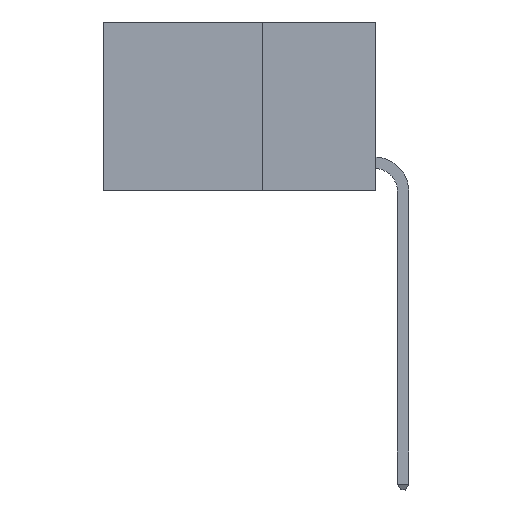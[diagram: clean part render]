
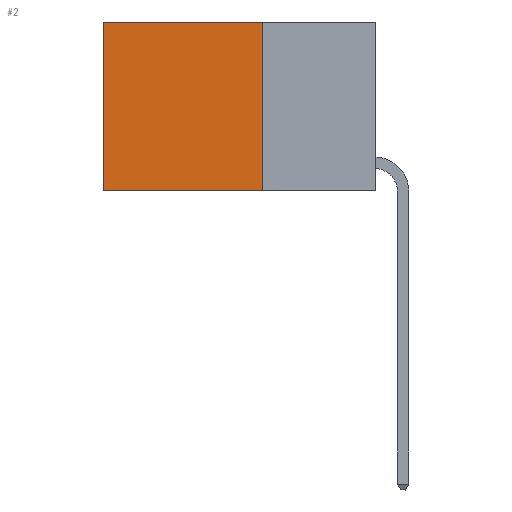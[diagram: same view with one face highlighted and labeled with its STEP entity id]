
A CAD part, left-side view. The second image highlights one B-rep face of the part: STEP entity #2.
In plain terms, the highlighted planar face has unit normal (-1, 0, 0).
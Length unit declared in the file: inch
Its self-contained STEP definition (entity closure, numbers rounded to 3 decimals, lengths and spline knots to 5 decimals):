
#2 = ADVANCED_FACE ( 'NONE', ( #24135 ), #3271, .F. ) ;
#2977 = EDGE_CURVE ( 'NONE', #5041, #15713, #22071, .T. ) ;
#3009 = EDGE_CURVE ( 'NONE', #5041, #8634, #20751, .T. ) ;
#3122 = CARTESIAN_POINT ( 'NONE',  ( 0.2625, 0.6, 0. ) ) ;
#3271 = PLANE ( 'NONE',  #3930 ) ;
#3333 = EDGE_LOOP ( 'NONE', ( #25702, #17631, #15450, #8585 ) ) ;
#3930 = AXIS2_PLACEMENT_3D ( 'NONE', #10370, #13940, #21242 ) ;
#5041 = VERTEX_POINT ( 'NONE', #12131 ) ;
#5551 = DIRECTION ( 'NONE',  ( 0., 1., 0. ) ) ;
#7100 = LINE ( 'NONE', #11531, #23403 ) ;
#8234 = DIRECTION ( 'NONE',  ( 0., 0., -1. ) ) ;
#8585 = ORIENTED_EDGE ( 'NONE', *, *, #3009, .T. ) ;
#8634 = VERTEX_POINT ( 'NONE', #14717 ) ;
#9954 = CARTESIAN_POINT ( 'NONE',  ( 0.2625, 0.6, -0.37 ) ) ;
#10370 = CARTESIAN_POINT ( 'NONE',  ( 0.2625, 0.25, 0. ) ) ;
#11531 = CARTESIAN_POINT ( 'NONE',  ( 0.2625, 0.25, -0.37 ) ) ;
#12131 = CARTESIAN_POINT ( 'NONE',  ( 0.2625, 0.25, 0. ) ) ;
#13940 = DIRECTION ( 'NONE',  ( 1., 0., 0. ) ) ;
#14717 = CARTESIAN_POINT ( 'NONE',  ( 0.2625, 0.6, 0. ) ) ;
#14762 = VECTOR ( 'NONE', #24476, 39.37008 ) ;
#15139 = VECTOR ( 'NONE', #5551, 39.37008 ) ;
#15450 = ORIENTED_EDGE ( 'NONE', *, *, #2977, .F. ) ;
#15713 = VERTEX_POINT ( 'NONE', #22586 ) ;
#16905 = EDGE_CURVE ( 'NONE', #15713, #17656, #7100, .T. ) ;
#17631 = ORIENTED_EDGE ( 'NONE', *, *, #16905, .F. ) ;
#17656 = VERTEX_POINT ( 'NONE', #9954 ) ;
#17834 = DIRECTION ( 'NONE',  ( 0., 1., 0. ) ) ;
#20751 = LINE ( 'NONE', #21615, #15139 ) ;
#21242 = DIRECTION ( 'NONE',  ( 0., 0., -1. ) ) ;
#21412 = CARTESIAN_POINT ( 'NONE',  ( 0.2625, 0.25, 0. ) ) ;
#21493 = VECTOR ( 'NONE', #8234, 39.37008 ) ;
#21615 = CARTESIAN_POINT ( 'NONE',  ( 0.2625, 0.25, 0. ) ) ;
#22071 = LINE ( 'NONE', #21412, #21493 ) ;
#22586 = CARTESIAN_POINT ( 'NONE',  ( 0.2625, 0.25, -0.37 ) ) ;
#23403 = VECTOR ( 'NONE', #17834, 39.37008 ) ;
#24135 = FACE_OUTER_BOUND ( 'NONE', #3333, .T. ) ;
#24476 = DIRECTION ( 'NONE',  ( 0., 0., -1. ) ) ;
#25702 = ORIENTED_EDGE ( 'NONE', *, *, #25943, .T. ) ;
#25943 = EDGE_CURVE ( 'NONE', #8634, #17656, #25975, .T. ) ;
#25975 = LINE ( 'NONE', #3122, #14762 ) ;
